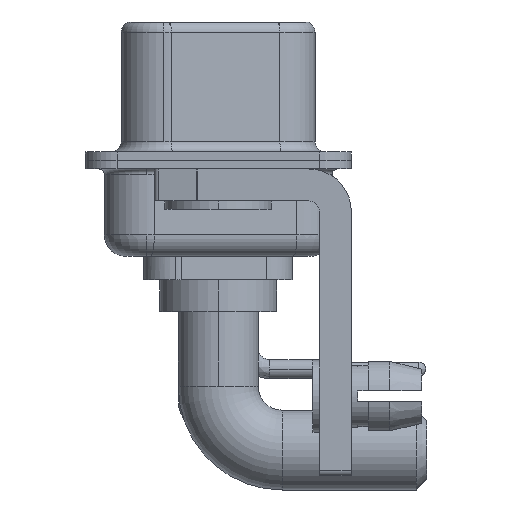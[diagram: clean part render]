
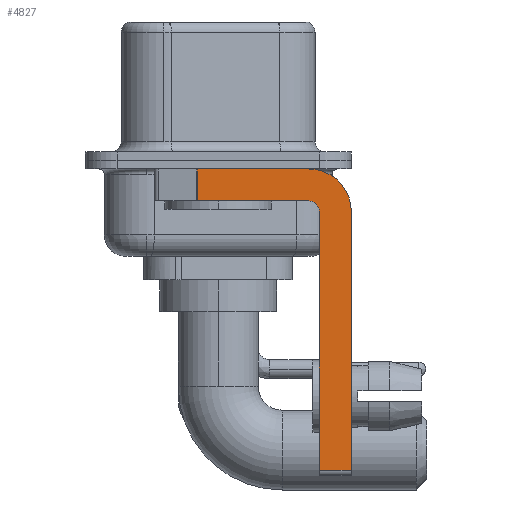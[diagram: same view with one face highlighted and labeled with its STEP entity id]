
A CAD part, left-side view. The second image highlights one B-rep face of the part: STEP entity #4827.
In plain terms, the highlighted planar face has unit normal (-1, 0, 0).
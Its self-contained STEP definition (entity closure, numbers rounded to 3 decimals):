
#114 = VERTEX_POINT ( 'NONE', #27137 ) ;
#285 = CARTESIAN_POINT ( 'NONE',  ( -2.9, -4.25, -0.4 ) ) ;
#663 = CARTESIAN_POINT ( 'NONE',  ( -2.9, 0.978, -1.9 ) ) ;
#1360 = AXIS2_PLACEMENT_3D ( 'NONE', #14523, #26862, #21719 ) ;
#1651 = EDGE_CURVE ( 'NONE', #25749, #13648, #23193, .T. ) ;
#2192 = ORIENTED_EDGE ( 'NONE', *, *, #15695, .F. ) ;
#2753 = LINE ( 'NONE', #24617, #12561 ) ;
#3083 = AXIS2_PLACEMENT_3D ( 'NONE', #4316, #25710, #21350 ) ;
#3114 = VECTOR ( 'NONE', #16484, 1000. ) ;
#3190 = DIRECTION ( 'NONE',  ( -1., 0., 0. ) ) ;
#3314 = VERTEX_POINT ( 'NONE', #8969 ) ;
#3410 = CARTESIAN_POINT ( 'NONE',  ( -2.9, -4.75, -14.55 ) ) ;
#4316 = CARTESIAN_POINT ( 'NONE',  ( -2.9, -4.25, -2.4 ) ) ;
#4783 = VERTEX_POINT ( 'NONE', #3410 ) ;
#4827 = ADVANCED_FACE ( 'NONE', ( #6672 ), #9163, .F. ) ;
#5124 = ORIENTED_EDGE ( 'NONE', *, *, #15651, .F. ) ;
#6245 = EDGE_CURVE ( 'NONE', #4783, #114, #2753, .T. ) ;
#6646 = CARTESIAN_POINT ( 'NONE',  ( -2.9, 3., -0.4 ) ) ;
#6672 = FACE_OUTER_BOUND ( 'NONE', #28838, .T. ) ;
#7208 = VECTOR ( 'NONE', #8260, 1000. ) ;
#7735 = DIRECTION ( 'NONE',  ( 0., 0., 1. ) ) ;
#7785 = CARTESIAN_POINT ( 'NONE',  ( -2.9, -4.25, -1.9 ) ) ;
#8207 = EDGE_CURVE ( 'NONE', #4783, #3314, #8409, .T. ) ;
#8260 = DIRECTION ( 'NONE',  ( 0., 0., 1. ) ) ;
#8409 = LINE ( 'NONE', #24647, #7208 ) ;
#8968 = ORIENTED_EDGE ( 'NONE', *, *, #6245, .T. ) ;
#8969 = CARTESIAN_POINT ( 'NONE',  ( -2.9, -4.75, -2.4 ) ) ;
#9163 = PLANE ( 'NONE',  #3083 ) ;
#9343 = EDGE_CURVE ( 'NONE', #25278, #13459, #23726, .T. ) ;
#10078 = CARTESIAN_POINT ( 'NONE',  ( -2.9, -6.25, -2.4 ) ) ;
#10501 = EDGE_CURVE ( 'NONE', #25749, #13459, #24726, .T. ) ;
#11404 = EDGE_CURVE ( 'NONE', #13648, #30562, #24316, .T. ) ;
#11972 = DIRECTION ( 'NONE',  ( 0., -1., 0. ) ) ;
#12561 = VECTOR ( 'NONE', #11972, 1000. ) ;
#13459 = VERTEX_POINT ( 'NONE', #28979 ) ;
#13648 = VERTEX_POINT ( 'NONE', #285 ) ;
#13876 = DIRECTION ( 'NONE',  ( 0., 1., 0. ) ) ;
#14523 = CARTESIAN_POINT ( 'NONE',  ( -2.9, -4.25, -2.4 ) ) ;
#15221 = DIRECTION ( 'NONE',  ( 0., 0., -1. ) ) ;
#15229 = ORIENTED_EDGE ( 'NONE', *, *, #10501, .T. ) ;
#15492 = CIRCLE ( 'NONE', #26988, 0.5 ) ;
#15651 = EDGE_CURVE ( 'NONE', #30562, #114, #22105, .T. ) ;
#15695 = EDGE_CURVE ( 'NONE', #3314, #25278, #15492, .T. ) ;
#16230 = CARTESIAN_POINT ( 'NONE',  ( -2.9, -4.25, -1.9 ) ) ;
#16484 = DIRECTION ( 'NONE',  ( 0., -1., 0. ) ) ;
#16820 = ORIENTED_EDGE ( 'NONE', *, *, #9343, .F. ) ;
#17106 = CARTESIAN_POINT ( 'NONE',  ( -2.9, -4.25, -2.4 ) ) ;
#17133 = ORIENTED_EDGE ( 'NONE', *, *, #8207, .F. ) ;
#19572 = CARTESIAN_POINT ( 'NONE',  ( -2.9, 0.978, -0.4 ) ) ;
#19708 = VECTOR ( 'NONE', #13876, 1000. ) ;
#21350 = DIRECTION ( 'NONE',  ( 0., 0., -1. ) ) ;
#21719 = DIRECTION ( 'NONE',  ( 0., 0., -1. ) ) ;
#22105 = LINE ( 'NONE', #22571, #25955 ) ;
#22571 = CARTESIAN_POINT ( 'NONE',  ( -2.9, -6.25, -2.4 ) ) ;
#23193 = LINE ( 'NONE', #6646, #3114 ) ;
#23726 = LINE ( 'NONE', #16230, #19708 ) ;
#24316 = CIRCLE ( 'NONE', #1360, 2. ) ;
#24617 = CARTESIAN_POINT ( 'NONE',  ( -2.9, -4.25, -14.55 ) ) ;
#24647 = CARTESIAN_POINT ( 'NONE',  ( -2.9, -4.75, -14.8 ) ) ;
#24726 = LINE ( 'NONE', #663, #25756 ) ;
#25278 = VERTEX_POINT ( 'NONE', #7785 ) ;
#25710 = DIRECTION ( 'NONE',  ( 1., 0., 0. ) ) ;
#25749 = VERTEX_POINT ( 'NONE', #19572 ) ;
#25756 = VECTOR ( 'NONE', #29432, 1000. ) ;
#25955 = VECTOR ( 'NONE', #15221, 1000. ) ;
#26070 = ORIENTED_EDGE ( 'NONE', *, *, #11404, .F. ) ;
#26862 = DIRECTION ( 'NONE',  ( 1., 0., 0. ) ) ;
#26988 = AXIS2_PLACEMENT_3D ( 'NONE', #17106, #3190, #7735 ) ;
#27137 = CARTESIAN_POINT ( 'NONE',  ( -2.9, -6.25, -14.55 ) ) ;
#28838 = EDGE_LOOP ( 'NONE', ( #30709, #15229, #16820, #2192, #17133, #8968, #5124, #26070 ) ) ;
#28979 = CARTESIAN_POINT ( 'NONE',  ( -2.9, 0.978, -1.9 ) ) ;
#29432 = DIRECTION ( 'NONE',  ( 0., 0., -1. ) ) ;
#30562 = VERTEX_POINT ( 'NONE', #10078 ) ;
#30709 = ORIENTED_EDGE ( 'NONE', *, *, #1651, .F. ) ;
